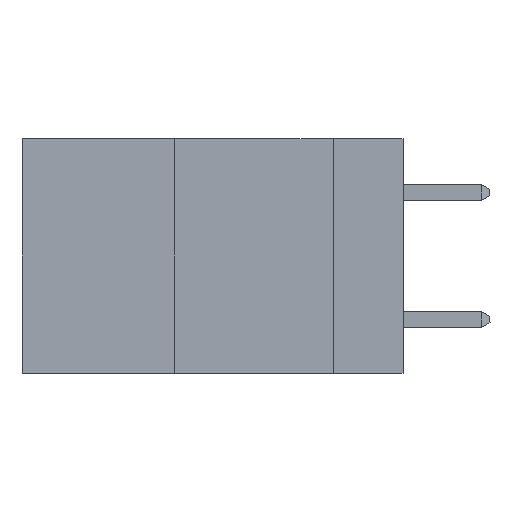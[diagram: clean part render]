
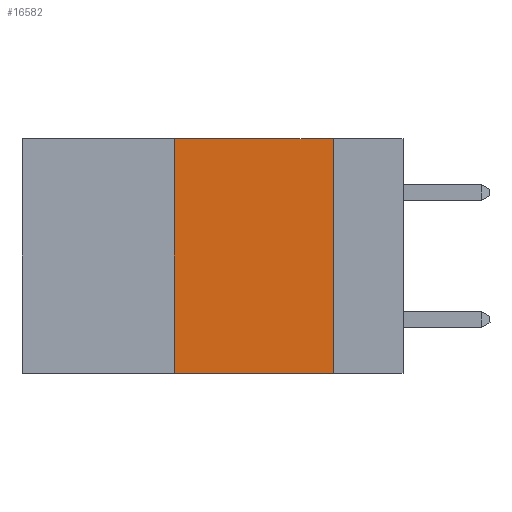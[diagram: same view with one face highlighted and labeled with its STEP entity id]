
A CAD part, left-side view. The second image highlights one B-rep face of the part: STEP entity #16582.
In plain terms, the highlighted planar face has unit normal (-1, 0, 0).
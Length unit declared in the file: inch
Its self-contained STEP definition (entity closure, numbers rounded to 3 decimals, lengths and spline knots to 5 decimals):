
#49 = VERTEX_POINT ( 'NONE', #2522 ) ;
#183 = DIRECTION ( 'NONE',  ( 0., 0., 1. ) ) ;
#2068 = EDGE_CURVE ( 'NONE', #16054, #12687, #5890, .T. ) ;
#2154 = EDGE_CURVE ( 'NONE', #9682, #49, #8156, .T. ) ;
#2299 = VECTOR ( 'NONE', #12243, 39.37008 ) ;
#2522 = CARTESIAN_POINT ( 'NONE',  ( 0., 0.11, -0.37 ) ) ;
#3308 = CARTESIAN_POINT ( 'NONE',  ( 0., 0.6, 0. ) ) ;
#4672 = VECTOR ( 'NONE', #11595, 39.37008 ) ;
#5890 = LINE ( 'NONE', #6225, #2299 ) ;
#5984 = DIRECTION ( 'NONE',  ( 0., 0., -1. ) ) ;
#6225 = CARTESIAN_POINT ( 'NONE',  ( 0., 0.6, 0. ) ) ;
#7058 = EDGE_LOOP ( 'NONE', ( #8297, #17284, #14573, #8955 ) ) ;
#7577 = EDGE_CURVE ( 'NONE', #12687, #49, #14393, .T. ) ;
#8156 = LINE ( 'NONE', #10935, #4672 ) ;
#8297 = ORIENTED_EDGE ( 'NONE', *, *, #7577, .F. ) ;
#8366 = CARTESIAN_POINT ( 'NONE',  ( 0., 0.36, -0.37 ) ) ;
#8427 = EDGE_CURVE ( 'NONE', #9682, #16054, #12932, .T. ) ;
#8955 = ORIENTED_EDGE ( 'NONE', *, *, #2154, .T. ) ;
#9007 = CARTESIAN_POINT ( 'NONE',  ( 0., 0.11, 0. ) ) ;
#9338 = VECTOR ( 'NONE', #183, 39.37008 ) ;
#9682 = VERTEX_POINT ( 'NONE', #8366 ) ;
#10812 = VECTOR ( 'NONE', #14257, 39.37008 ) ;
#10935 = CARTESIAN_POINT ( 'NONE',  ( 0., 0.6, -0.37 ) ) ;
#11056 = CARTESIAN_POINT ( 'NONE',  ( 0., 0.36, 0. ) ) ;
#11299 = CARTESIAN_POINT ( 'NONE',  ( 0., 0.36, 0. ) ) ;
#11595 = DIRECTION ( 'NONE',  ( 0., -1., 0. ) ) ;
#12243 = DIRECTION ( 'NONE',  ( 0., -1., 0. ) ) ;
#12658 = PLANE ( 'NONE',  #15334 ) ;
#12687 = VERTEX_POINT ( 'NONE', #9007 ) ;
#12925 = CARTESIAN_POINT ( 'NONE',  ( 0., 0.11, 0. ) ) ;
#12932 = LINE ( 'NONE', #11056, #9338 ) ;
#13982 = DIRECTION ( 'NONE',  ( 1., 0., 0. ) ) ;
#14257 = DIRECTION ( 'NONE',  ( 0., 0., -1. ) ) ;
#14393 = LINE ( 'NONE', #12925, #10812 ) ;
#14573 = ORIENTED_EDGE ( 'NONE', *, *, #8427, .F. ) ;
#15334 = AXIS2_PLACEMENT_3D ( 'NONE', #3308, #13982, #5984 ) ;
#16054 = VERTEX_POINT ( 'NONE', #11299 ) ;
#16582 = ADVANCED_FACE ( 'NONE', ( #16626 ), #12658, .F. ) ;
#16626 = FACE_OUTER_BOUND ( 'NONE', #7058, .T. ) ;
#17284 = ORIENTED_EDGE ( 'NONE', *, *, #2068, .F. ) ;
